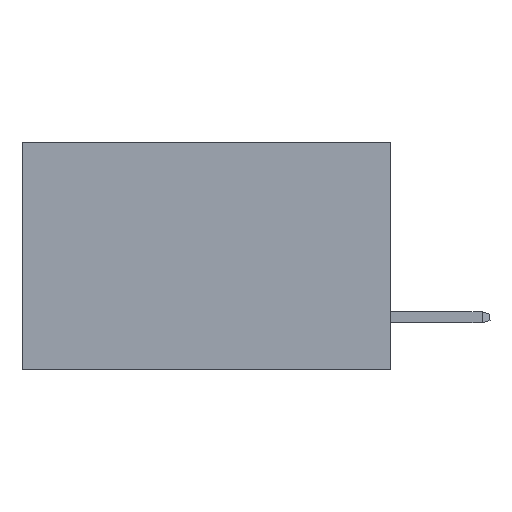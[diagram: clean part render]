
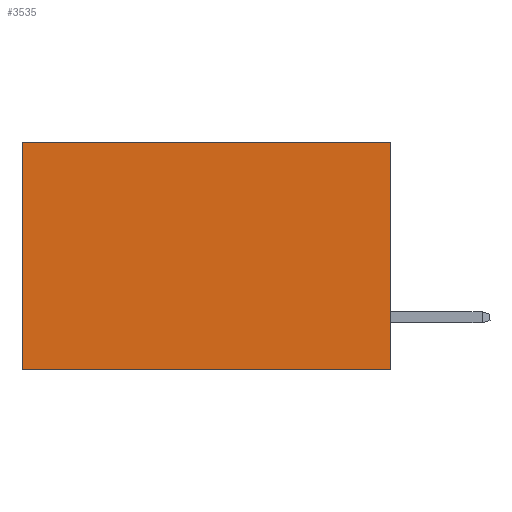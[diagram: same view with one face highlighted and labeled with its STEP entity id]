
A CAD part, left-side view. The second image highlights one B-rep face of the part: STEP entity #3535.
In plain terms, the highlighted planar face has unit normal (-1, 0, 0).
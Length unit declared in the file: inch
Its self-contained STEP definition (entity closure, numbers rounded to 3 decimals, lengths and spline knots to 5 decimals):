
#492 = DIRECTION ( 'NONE',  ( 0., 1., 0. ) ) ;
#1016 = CARTESIAN_POINT ( 'NONE',  ( 0.2875, 0.6, 0. ) ) ;
#1665 = EDGE_CURVE ( 'NONE', #6052, #4413, #1672, .T. ) ;
#1672 = LINE ( 'NONE', #4986, #6431 ) ;
#2115 = CARTESIAN_POINT ( 'NONE',  ( 0.2875, 0.6, -0.37 ) ) ;
#2303 = ORIENTED_EDGE ( 'NONE', *, *, #1665, .T. ) ;
#2458 = VERTEX_POINT ( 'NONE', #5804 ) ;
#2620 = ORIENTED_EDGE ( 'NONE', *, *, #7161, .T. ) ;
#2986 = DIRECTION ( 'NONE',  ( 0., 0., -1. ) ) ;
#3214 = EDGE_LOOP ( 'NONE', ( #2303, #7617, #5408, #2620 ) ) ;
#3256 = EDGE_CURVE ( 'NONE', #5353, #2458, #8409, .T. ) ;
#3535 = ADVANCED_FACE ( 'NONE', ( #4949 ), #4560, .F. ) ;
#4060 = CARTESIAN_POINT ( 'NONE',  ( 0.2875, 0., -0.37 ) ) ;
#4319 = VECTOR ( 'NONE', #492, 39.37008 ) ;
#4413 = VERTEX_POINT ( 'NONE', #2115 ) ;
#4442 = DIRECTION ( 'NONE',  ( 1., 0., 0. ) ) ;
#4560 = PLANE ( 'NONE',  #8366 ) ;
#4949 = FACE_OUTER_BOUND ( 'NONE', #3214, .T. ) ;
#4986 = CARTESIAN_POINT ( 'NONE',  ( 0.2875, 0.6, 0. ) ) ;
#5179 = CARTESIAN_POINT ( 'NONE',  ( 0.2875, 0., 0. ) ) ;
#5353 = VERTEX_POINT ( 'NONE', #8705 ) ;
#5408 = ORIENTED_EDGE ( 'NONE', *, *, #3256, .F. ) ;
#5804 = CARTESIAN_POINT ( 'NONE',  ( 0.2875, 0., -0.37 ) ) ;
#6052 = VERTEX_POINT ( 'NONE', #1016 ) ;
#6178 = CARTESIAN_POINT ( 'NONE',  ( 0.2875, 0., 0. ) ) ;
#6352 = DIRECTION ( 'NONE',  ( 0., 0., -1. ) ) ;
#6427 = VECTOR ( 'NONE', #6475, 39.37008 ) ;
#6431 = VECTOR ( 'NONE', #6352, 39.37008 ) ;
#6475 = DIRECTION ( 'NONE',  ( 0., 1., 0. ) ) ;
#7161 = EDGE_CURVE ( 'NONE', #5353, #6052, #8230, .T. ) ;
#7529 = LINE ( 'NONE', #4060, #4319 ) ;
#7617 = ORIENTED_EDGE ( 'NONE', *, *, #8379, .F. ) ;
#8105 = DIRECTION ( 'NONE',  ( 0., 0., -1. ) ) ;
#8230 = LINE ( 'NONE', #6178, #6427 ) ;
#8366 = AXIS2_PLACEMENT_3D ( 'NONE', #8699, #4442, #8105 ) ;
#8379 = EDGE_CURVE ( 'NONE', #2458, #4413, #7529, .T. ) ;
#8409 = LINE ( 'NONE', #5179, #8929 ) ;
#8699 = CARTESIAN_POINT ( 'NONE',  ( 0.2875, 0., 0. ) ) ;
#8705 = CARTESIAN_POINT ( 'NONE',  ( 0.2875, 0., 0. ) ) ;
#8929 = VECTOR ( 'NONE', #2986, 39.37008 ) ;
